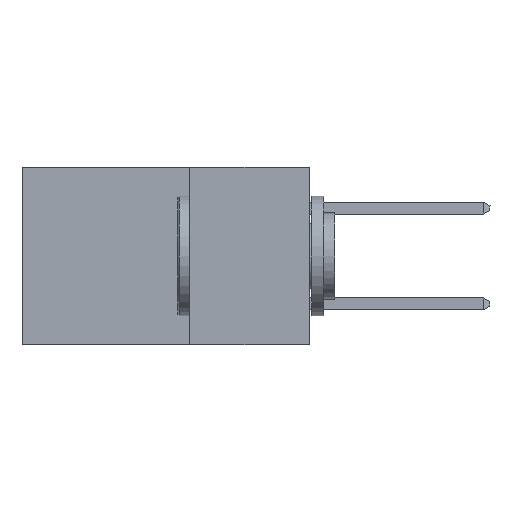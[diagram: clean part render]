
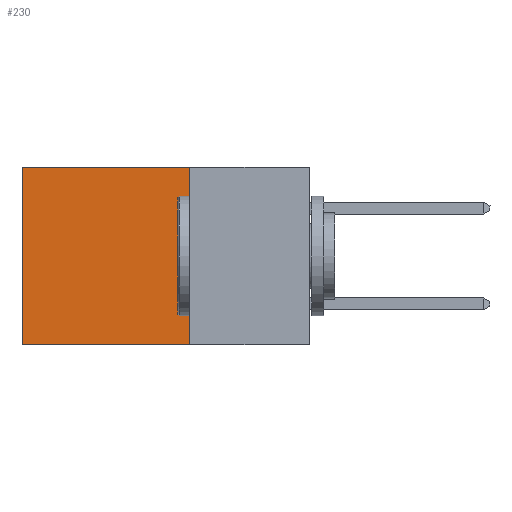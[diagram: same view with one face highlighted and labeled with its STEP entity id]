
A CAD part, left-side view. The second image highlights one B-rep face of the part: STEP entity #230.
In plain terms, the highlighted planar face has unit normal (-1, 0, 0).
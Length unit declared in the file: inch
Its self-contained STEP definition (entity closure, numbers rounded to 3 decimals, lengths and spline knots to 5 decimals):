
#230 = ADVANCED_FACE ( 'NONE', ( #4925 ), #6394, .F. ) ;
#340 = CARTESIAN_POINT ( 'NONE',  ( 0.2875, 0.6, 0. ) ) ;
#879 = ORIENTED_EDGE ( 'NONE', *, *, #10736, .T. ) ;
#1157 = CARTESIAN_POINT ( 'NONE',  ( 0.2875, 0.25, 0. ) ) ;
#1214 = CARTESIAN_POINT ( 'NONE',  ( 0.2875, 0.25, 0. ) ) ;
#1220 = CARTESIAN_POINT ( 'NONE',  ( 0.2875, 0.25, 0. ) ) ;
#2099 = EDGE_LOOP ( 'NONE', ( #879, #10416, #2220, #9284 ) ) ;
#2220 = ORIENTED_EDGE ( 'NONE', *, *, #7964, .F. ) ;
#2305 = DIRECTION ( 'NONE',  ( 0., 0., -1. ) ) ;
#2531 = AXIS2_PLACEMENT_3D ( 'NONE', #1157, #6133, #6436 ) ;
#3257 = EDGE_CURVE ( 'NONE', #11104, #8125, #4698, .T. ) ;
#3264 = DIRECTION ( 'NONE',  ( 0., 1., 0. ) ) ;
#3354 = LINE ( 'NONE', #9555, #7567 ) ;
#3413 = CARTESIAN_POINT ( 'NONE',  ( 0.2875, 0.6, -0.37 ) ) ;
#3968 = CARTESIAN_POINT ( 'NONE',  ( 0.2875, 0.6, 0. ) ) ;
#4491 = LINE ( 'NONE', #1220, #9325 ) ;
#4698 = LINE ( 'NONE', #1214, #7362 ) ;
#4925 = FACE_OUTER_BOUND ( 'NONE', #2099, .T. ) ;
#5591 = LINE ( 'NONE', #3968, #9765 ) ;
#6133 = DIRECTION ( 'NONE',  ( 1., 0., 0. ) ) ;
#6220 = EDGE_CURVE ( 'NONE', #6514, #10958, #3354, .T. ) ;
#6394 = PLANE ( 'NONE',  #2531 ) ;
#6436 = DIRECTION ( 'NONE',  ( 0., 0., -1. ) ) ;
#6514 = VERTEX_POINT ( 'NONE', #10512 ) ;
#7362 = VECTOR ( 'NONE', #3264, 39.37008 ) ;
#7567 = VECTOR ( 'NONE', #10323, 39.37008 ) ;
#7964 = EDGE_CURVE ( 'NONE', #11104, #6514, #4491, .T. ) ;
#8125 = VERTEX_POINT ( 'NONE', #340 ) ;
#8859 = CARTESIAN_POINT ( 'NONE',  ( 0.2875, 0.25, 0. ) ) ;
#9284 = ORIENTED_EDGE ( 'NONE', *, *, #3257, .T. ) ;
#9325 = VECTOR ( 'NONE', #2305, 39.37008 ) ;
#9555 = CARTESIAN_POINT ( 'NONE',  ( 0.2875, 0.25, -0.37 ) ) ;
#9765 = VECTOR ( 'NONE', #11527, 39.37008 ) ;
#10323 = DIRECTION ( 'NONE',  ( 0., 1., 0. ) ) ;
#10416 = ORIENTED_EDGE ( 'NONE', *, *, #6220, .F. ) ;
#10512 = CARTESIAN_POINT ( 'NONE',  ( 0.2875, 0.25, -0.37 ) ) ;
#10736 = EDGE_CURVE ( 'NONE', #8125, #10958, #5591, .T. ) ;
#10958 = VERTEX_POINT ( 'NONE', #3413 ) ;
#11104 = VERTEX_POINT ( 'NONE', #8859 ) ;
#11527 = DIRECTION ( 'NONE',  ( 0., 0., -1. ) ) ;
